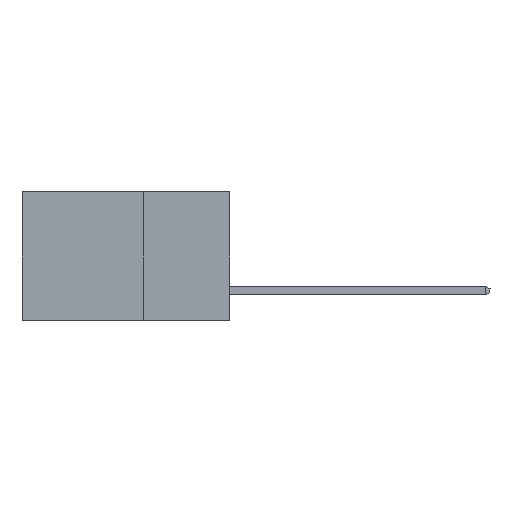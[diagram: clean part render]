
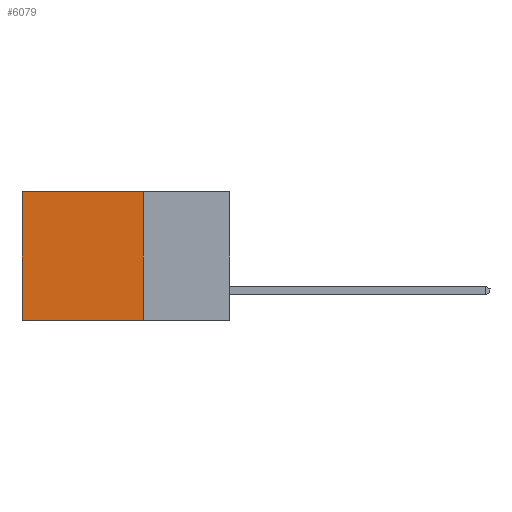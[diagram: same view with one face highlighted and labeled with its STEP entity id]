
A CAD part, left-side view. The second image highlights one B-rep face of the part: STEP entity #6079.
In plain terms, the highlighted planar face has unit normal (-1, 0, 0).
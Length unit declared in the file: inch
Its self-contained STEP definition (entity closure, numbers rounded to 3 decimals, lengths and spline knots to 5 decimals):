
#26 = CARTESIAN_POINT ( 'NONE',  ( 0.2615, 0.25, -0.37 ) ) ;
#120 = EDGE_CURVE ( 'NONE', #1386, #10328, #5550, .T. ) ;
#194 = EDGE_CURVE ( 'NONE', #1401, #5936, #4162, .T. ) ;
#430 = VECTOR ( 'NONE', #7607, 39.37008 ) ;
#696 = DIRECTION ( 'NONE',  ( 0., 0., -1. ) ) ;
#1386 = VERTEX_POINT ( 'NONE', #10637 ) ;
#1401 = VERTEX_POINT ( 'NONE', #9766 ) ;
#2080 = DIRECTION ( 'NONE',  ( 0., 1., 0. ) ) ;
#2139 = DIRECTION ( 'NONE',  ( 0., 1., 0. ) ) ;
#2405 = CARTESIAN_POINT ( 'NONE',  ( 0.2615, 0.6, 0. ) ) ;
#2590 = ORIENTED_EDGE ( 'NONE', *, *, #194, .F. ) ;
#2749 = DIRECTION ( 'NONE',  ( 1., 0., 0. ) ) ;
#2921 = PLANE ( 'NONE',  #9759 ) ;
#3177 = LINE ( 'NONE', #10364, #9550 ) ;
#3481 = ORIENTED_EDGE ( 'NONE', *, *, #4323, .T. ) ;
#3763 = EDGE_LOOP ( 'NONE', ( #3481, #2590, #8380, #6441 ) ) ;
#4068 = CARTESIAN_POINT ( 'NONE',  ( 0.2615, 0.6, -0.37 ) ) ;
#4162 = LINE ( 'NONE', #7533, #5613 ) ;
#4180 = LINE ( 'NONE', #4068, #430 ) ;
#4323 = EDGE_CURVE ( 'NONE', #10328, #5936, #4180, .T. ) ;
#4867 = VECTOR ( 'NONE', #2080, 39.37008 ) ;
#5550 = LINE ( 'NONE', #10913, #4867 ) ;
#5613 = VECTOR ( 'NONE', #2139, 39.37008 ) ;
#5936 = VERTEX_POINT ( 'NONE', #8614 ) ;
#6079 = ADVANCED_FACE ( 'NONE', ( #8021 ), #2921, .F. ) ;
#6441 = ORIENTED_EDGE ( 'NONE', *, *, #120, .T. ) ;
#7533 = CARTESIAN_POINT ( 'NONE',  ( 0.2615, 0.25, -0.37 ) ) ;
#7607 = DIRECTION ( 'NONE',  ( 0., 0., -1. ) ) ;
#8021 = FACE_OUTER_BOUND ( 'NONE', #3763, .T. ) ;
#8380 = ORIENTED_EDGE ( 'NONE', *, *, #11236, .F. ) ;
#8614 = CARTESIAN_POINT ( 'NONE',  ( 0.2615, 0.6, -0.37 ) ) ;
#9550 = VECTOR ( 'NONE', #696, 39.37008 ) ;
#9759 = AXIS2_PLACEMENT_3D ( 'NONE', #26, #2749, #9821 ) ;
#9766 = CARTESIAN_POINT ( 'NONE',  ( 0.2615, 0.25, -0.37 ) ) ;
#9821 = DIRECTION ( 'NONE',  ( 0., 0., -1. ) ) ;
#10328 = VERTEX_POINT ( 'NONE', #2405 ) ;
#10364 = CARTESIAN_POINT ( 'NONE',  ( 0.2615, 0.25, -0.37 ) ) ;
#10637 = CARTESIAN_POINT ( 'NONE',  ( 0.2615, 0.25, 0. ) ) ;
#10913 = CARTESIAN_POINT ( 'NONE',  ( 0.2615, 0.25, 0. ) ) ;
#11236 = EDGE_CURVE ( 'NONE', #1386, #1401, #3177, .T. ) ;
